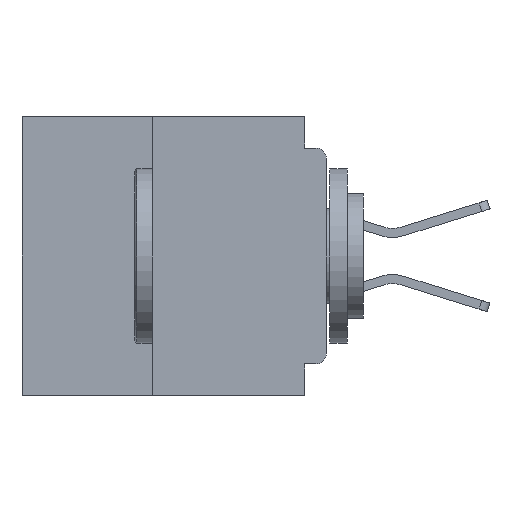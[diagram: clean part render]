
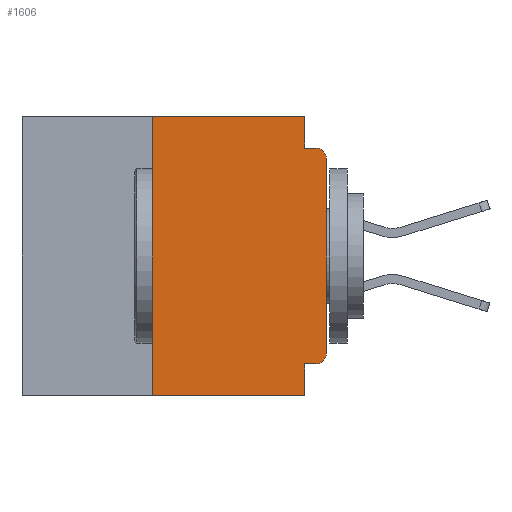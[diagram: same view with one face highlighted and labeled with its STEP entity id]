
A CAD part, left-side view. The second image highlights one B-rep face of the part: STEP entity #1606.
In plain terms, the highlighted planar face has unit normal (-1, 0, 0).
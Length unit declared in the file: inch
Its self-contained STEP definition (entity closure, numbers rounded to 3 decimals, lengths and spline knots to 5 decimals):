
#10 = EDGE_CURVE ( 'NONE', #18310, #26327, #28934, .T. ) ;
#1283 = DIRECTION ( 'NONE',  ( 0., -1., 0. ) ) ;
#1606 = ADVANCED_FACE ( 'NONE', ( #47589 ), #45662, .F. ) ;
#1762 = EDGE_LOOP ( 'NONE', ( #18512, #38045, #41454, #44855, #28881, #10474, #32330, #23730, #43163, #8083 ) ) ;
#1936 = VERTEX_POINT ( 'NONE', #15718 ) ;
#2976 = CARTESIAN_POINT ( 'NONE',  ( 0., 0.437, 0. ) ) ;
#3483 = AXIS2_PLACEMENT_3D ( 'NONE', #47732, #25867, #3708 ) ;
#3584 = VECTOR ( 'NONE', #1283, 39.37008 ) ;
#3664 = DIRECTION ( 'NONE',  ( 0., 0., -1. ) ) ;
#3708 = DIRECTION ( 'NONE',  ( 0., 0., -1. ) ) ;
#3914 = LINE ( 'NONE', #23047, #40767 ) ;
#3942 = DIRECTION ( 'NONE',  ( 0., 0., 1. ) ) ;
#5939 = VECTOR ( 'NONE', #14238, 39.37008 ) ;
#6207 = LINE ( 'NONE', #11530, #25834 ) ;
#7215 = VERTEX_POINT ( 'NONE', #32277 ) ;
#7590 = EDGE_CURVE ( 'NONE', #30136, #42113, #40422, .T. ) ;
#7995 = VERTEX_POINT ( 'NONE', #11824 ) ;
#8083 = ORIENTED_EDGE ( 'NONE', *, *, #15401, .T. ) ;
#8925 = CARTESIAN_POINT ( 'NONE',  ( 0., 0.031, 0. ) ) ;
#9460 = LINE ( 'NONE', #27114, #27911 ) ;
#9816 = CARTESIAN_POINT ( 'NONE',  ( 0., 0.25, 0. ) ) ;
#9841 = VERTEX_POINT ( 'NONE', #37167 ) ;
#10474 = ORIENTED_EDGE ( 'NONE', *, *, #10, .F. ) ;
#11175 = VECTOR ( 'NONE', #23739, 39.37008 ) ;
#11530 = CARTESIAN_POINT ( 'NONE',  ( 0., 0.437, -0.4 ) ) ;
#11824 = CARTESIAN_POINT ( 'NONE',  ( 0., 0.015, -0.045 ) ) ;
#13429 = CIRCLE ( 'NONE', #42223, 0.015 ) ;
#13551 = CARTESIAN_POINT ( 'NONE',  ( 0., 0.015, -0.355 ) ) ;
#14238 = DIRECTION ( 'NONE',  ( 0., -1., 0. ) ) ;
#14465 = EDGE_CURVE ( 'NONE', #42113, #7995, #15852, .T. ) ;
#15401 = EDGE_CURVE ( 'NONE', #16958, #37733, #13429, .T. ) ;
#15718 = CARTESIAN_POINT ( 'NONE',  ( 0., 0.031, -0.355 ) ) ;
#15852 = LINE ( 'NONE', #34261, #3584 ) ;
#16958 = VERTEX_POINT ( 'NONE', #13551 ) ;
#17875 = DIRECTION ( 'NONE',  ( 0., 0., -1. ) ) ;
#18310 = VERTEX_POINT ( 'NONE', #46704 ) ;
#18512 = ORIENTED_EDGE ( 'NONE', *, *, #41507, .T. ) ;
#21870 = CARTESIAN_POINT ( 'NONE',  ( 0., 0.031, 0. ) ) ;
#22832 = VECTOR ( 'NONE', #17875, 39.37008 ) ;
#23047 = CARTESIAN_POINT ( 'NONE',  ( 0., 0., -0.355 ) ) ;
#23730 = ORIENTED_EDGE ( 'NONE', *, *, #40507, .F. ) ;
#23739 = DIRECTION ( 'NONE',  ( 0., 0., -1. ) ) ;
#25587 = LINE ( 'NONE', #2976, #5939 ) ;
#25834 = VECTOR ( 'NONE', #37229, 39.37008 ) ;
#25835 = DIRECTION ( 'NONE',  ( -1., 0., 0. ) ) ;
#25867 = DIRECTION ( 'NONE',  ( -1., 0., 0. ) ) ;
#26020 = CARTESIAN_POINT ( 'NONE',  ( 0., 0.031, -0.045 ) ) ;
#26327 = VERTEX_POINT ( 'NONE', #9816 ) ;
#26744 = DIRECTION ( 'NONE',  ( 0., 1., 0. ) ) ;
#27114 = CARTESIAN_POINT ( 'NONE',  ( 0., 0., 0. ) ) ;
#27911 = VECTOR ( 'NONE', #30807, 39.37008 ) ;
#28881 = ORIENTED_EDGE ( 'NONE', *, *, #34367, .F. ) ;
#28934 = LINE ( 'NONE', #33824, #47172 ) ;
#30136 = VERTEX_POINT ( 'NONE', #21870 ) ;
#30188 = EDGE_CURVE ( 'NONE', #7215, #7995, #45486, .T. ) ;
#30807 = DIRECTION ( 'NONE',  ( 0., 0., 1. ) ) ;
#32277 = CARTESIAN_POINT ( 'NONE',  ( 0., 0., -0.06 ) ) ;
#32330 = ORIENTED_EDGE ( 'NONE', *, *, #45402, .T. ) ;
#32578 = LINE ( 'NONE', #39810, #22832 ) ;
#33824 = CARTESIAN_POINT ( 'NONE',  ( 0., 0.25, -0.4 ) ) ;
#34261 = CARTESIAN_POINT ( 'NONE',  ( 0., 0., -0.045 ) ) ;
#34367 = EDGE_CURVE ( 'NONE', #26327, #30136, #25587, .T. ) ;
#35369 = AXIS2_PLACEMENT_3D ( 'NONE', #43664, #41031, #40963 ) ;
#37167 = CARTESIAN_POINT ( 'NONE',  ( 0., 0.031, -0.4 ) ) ;
#37229 = DIRECTION ( 'NONE',  ( 0., -1., 0. ) ) ;
#37544 = EDGE_CURVE ( 'NONE', #16958, #1936, #3914, .T. ) ;
#37733 = VERTEX_POINT ( 'NONE', #42372 ) ;
#38045 = ORIENTED_EDGE ( 'NONE', *, *, #30188, .T. ) ;
#39810 = CARTESIAN_POINT ( 'NONE',  ( 0., 0.031, -0.4 ) ) ;
#40422 = LINE ( 'NONE', #8925, #11175 ) ;
#40507 = EDGE_CURVE ( 'NONE', #1936, #9841, #32578, .T. ) ;
#40767 = VECTOR ( 'NONE', #26744, 39.37008 ) ;
#40963 = DIRECTION ( 'NONE',  ( 0., 0., -1. ) ) ;
#41031 = DIRECTION ( 'NONE',  ( 1., 0., 0. ) ) ;
#41454 = ORIENTED_EDGE ( 'NONE', *, *, #14465, .F. ) ;
#41507 = EDGE_CURVE ( 'NONE', #37733, #7215, #9460, .T. ) ;
#42113 = VERTEX_POINT ( 'NONE', #26020 ) ;
#42223 = AXIS2_PLACEMENT_3D ( 'NONE', #47690, #25835, #3664 ) ;
#42372 = CARTESIAN_POINT ( 'NONE',  ( 0., 0., -0.34 ) ) ;
#43163 = ORIENTED_EDGE ( 'NONE', *, *, #37544, .F. ) ;
#43664 = CARTESIAN_POINT ( 'NONE',  ( 0., 0.437, 0. ) ) ;
#44855 = ORIENTED_EDGE ( 'NONE', *, *, #7590, .F. ) ;
#45402 = EDGE_CURVE ( 'NONE', #18310, #9841, #6207, .T. ) ;
#45486 = CIRCLE ( 'NONE', #3483, 0.015 ) ;
#45662 = PLANE ( 'NONE',  #35369 ) ;
#46704 = CARTESIAN_POINT ( 'NONE',  ( 0., 0.25, -0.4 ) ) ;
#47172 = VECTOR ( 'NONE', #3942, 39.37008 ) ;
#47589 = FACE_OUTER_BOUND ( 'NONE', #1762, .T. ) ;
#47690 = CARTESIAN_POINT ( 'NONE',  ( 0., 0.015, -0.34 ) ) ;
#47732 = CARTESIAN_POINT ( 'NONE',  ( 0., 0.015, -0.06 ) ) ;
